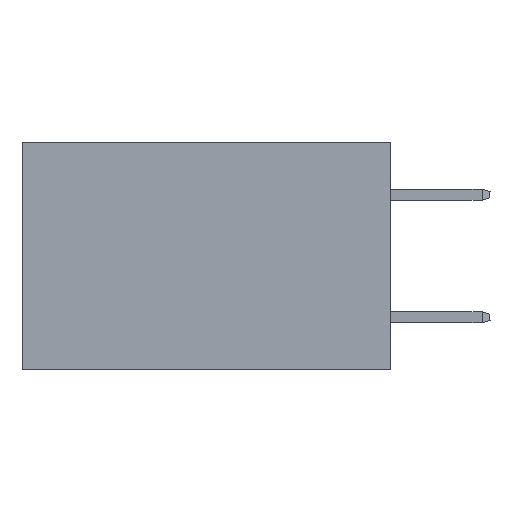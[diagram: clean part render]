
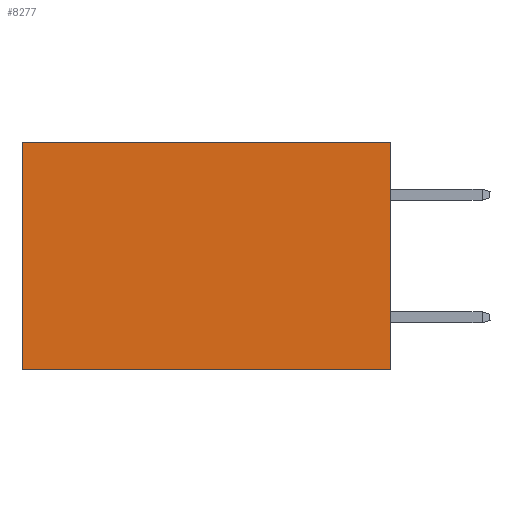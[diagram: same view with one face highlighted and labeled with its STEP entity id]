
A CAD part, left-side view. The second image highlights one B-rep face of the part: STEP entity #8277.
In plain terms, the highlighted planar face has unit normal (-1, 0, 0).
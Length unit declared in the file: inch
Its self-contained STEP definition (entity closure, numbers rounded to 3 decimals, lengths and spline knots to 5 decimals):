
#181 = FACE_OUTER_BOUND ( 'NONE', #1636, .T. ) ;
#273 = CARTESIAN_POINT ( 'NONE',  ( 0.2875, 0.6, -0.37 ) ) ;
#361 = CARTESIAN_POINT ( 'NONE',  ( 0.2875, 0., 0. ) ) ;
#1198 = DIRECTION ( 'NONE',  ( 1., 0., 0. ) ) ;
#1496 = VERTEX_POINT ( 'NONE', #273 ) ;
#1636 = EDGE_LOOP ( 'NONE', ( #9821, #9683, #5180, #2804 ) ) ;
#1667 = CARTESIAN_POINT ( 'NONE',  ( 0.2875, 0., 0. ) ) ;
#2721 = DIRECTION ( 'NONE',  ( 0., 1., 0. ) ) ;
#2804 = ORIENTED_EDGE ( 'NONE', *, *, #11228, .T. ) ;
#2938 = VERTEX_POINT ( 'NONE', #361 ) ;
#3210 = EDGE_CURVE ( 'NONE', #2938, #5113, #4110, .T. ) ;
#3740 = CARTESIAN_POINT ( 'NONE',  ( 0.2875, 0., 0. ) ) ;
#4110 = LINE ( 'NONE', #7092, #6171 ) ;
#4165 = CARTESIAN_POINT ( 'NONE',  ( 0.2875, 0.6, 0. ) ) ;
#4231 = VERTEX_POINT ( 'NONE', #10460 ) ;
#4402 = CARTESIAN_POINT ( 'NONE',  ( 0.2875, 0., -0.37 ) ) ;
#4481 = LINE ( 'NONE', #8792, #6812 ) ;
#5098 = DIRECTION ( 'NONE',  ( 0., 0., -1. ) ) ;
#5113 = VERTEX_POINT ( 'NONE', #4402 ) ;
#5180 = ORIENTED_EDGE ( 'NONE', *, *, #3210, .F. ) ;
#5548 = VECTOR ( 'NONE', #10319, 39.37008 ) ;
#5583 = EDGE_CURVE ( 'NONE', #4231, #1496, #5665, .T. ) ;
#5665 = LINE ( 'NONE', #4165, #9636 ) ;
#6171 = VECTOR ( 'NONE', #8103, 39.37008 ) ;
#6396 = PLANE ( 'NONE',  #6713 ) ;
#6713 = AXIS2_PLACEMENT_3D ( 'NONE', #3740, #1198, #7401 ) ;
#6812 = VECTOR ( 'NONE', #2721, 39.37008 ) ;
#7092 = CARTESIAN_POINT ( 'NONE',  ( 0.2875, 0., 0. ) ) ;
#7401 = DIRECTION ( 'NONE',  ( 0., 0., -1. ) ) ;
#8103 = DIRECTION ( 'NONE',  ( 0., 0., -1. ) ) ;
#8277 = ADVANCED_FACE ( 'NONE', ( #181 ), #6396, .F. ) ;
#8719 = EDGE_CURVE ( 'NONE', #5113, #1496, #4481, .T. ) ;
#8792 = CARTESIAN_POINT ( 'NONE',  ( 0.2875, 0., -0.37 ) ) ;
#9636 = VECTOR ( 'NONE', #5098, 39.37008 ) ;
#9683 = ORIENTED_EDGE ( 'NONE', *, *, #8719, .F. ) ;
#9821 = ORIENTED_EDGE ( 'NONE', *, *, #5583, .T. ) ;
#10307 = LINE ( 'NONE', #1667, #5548 ) ;
#10319 = DIRECTION ( 'NONE',  ( 0., 1., 0. ) ) ;
#10460 = CARTESIAN_POINT ( 'NONE',  ( 0.2875, 0.6, 0. ) ) ;
#11228 = EDGE_CURVE ( 'NONE', #2938, #4231, #10307, .T. ) ;
